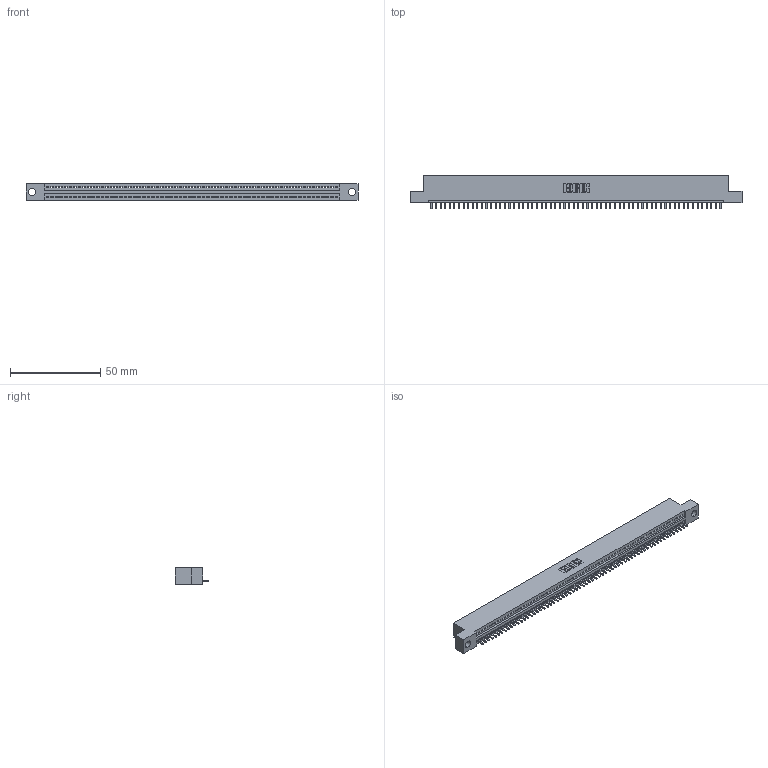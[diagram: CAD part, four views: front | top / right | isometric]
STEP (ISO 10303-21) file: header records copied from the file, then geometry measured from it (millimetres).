
FILE_DESCRIPTION (( 'STEP AP203' ), '1' );
FILE_NAME ('345-064-521-104.STEP', '2021-05-28T16:00:09', ( '' ), ( '' ), 'SwSTEP 2.0', 'SolidWorks 2020', '' );
FILE_SCHEMA (( 'CONFIG_CONTROL_DESIGN' ));
Length unit declared in the file: inch
Products named in the file (3): 345-292-001_345-293-121; 345-064-521-104; 345 Part_Flush Mounting Lugs - 0.156 Dia-TI
Assembly tree (65 placements, depth 2):
  345-064-521-104
    345 Part_Flush Mounting Lugs - 0.156 Dia-TI
    345-292-001_345-293-121  x64
Bounding box: 183.77 x 18.72 x 9.4 mm (x, y, z)
Volume: 17346.8 mm3; surface area: 22481.6 mm2
Topology: 65 solids, 65 shells, 3852 faces, 11641 edges, 7674 vertices
Faces by surface type: plane 2654, cylinder 1198
Entity records: 45643 total; most frequent: CARTESIAN_POINT 7914, ORIENTED_EDGE 7910, DIRECTION 6879, EDGE_CURVE 3955, VECTOR 3567, LINE 3567, VERTEX_POINT 2634, AXIS2_PLACEMENT_3D 1656
